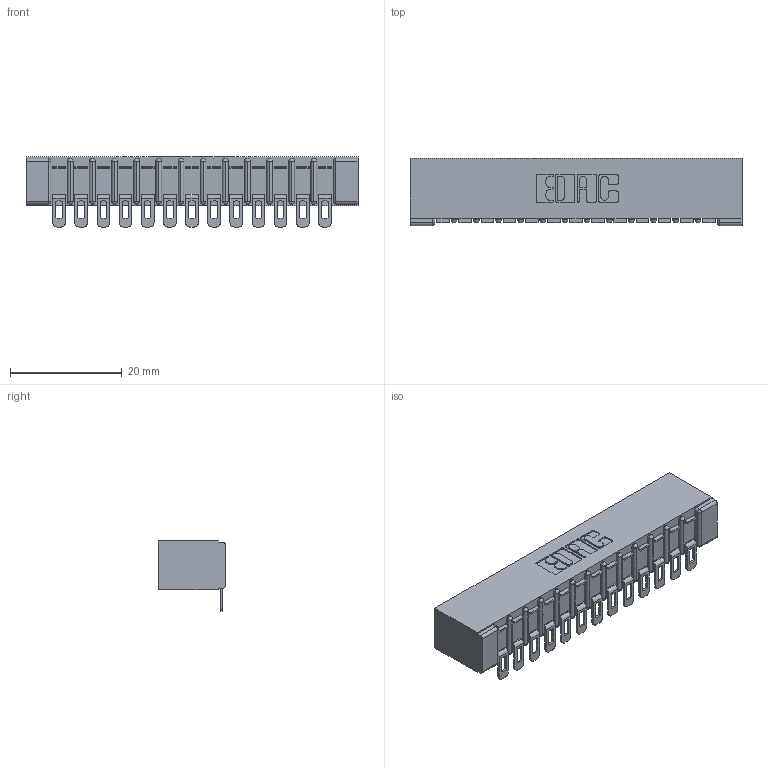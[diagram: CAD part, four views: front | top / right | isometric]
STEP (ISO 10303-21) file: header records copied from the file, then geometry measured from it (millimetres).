
FILE_DESCRIPTION (( 'STEP AP203' ), '1' );
FILE_NAME ('307-013-554-101.STEP', '2018-08-03T00:08:36', ( '' ), ( '' ), 'SwSTEP 2.0', 'SolidWorks 2016', '' );
FILE_SCHEMA (( 'CONFIG_CONTROL_DESIGN' ));
Length unit declared in the file: inch
Products named in the file (3): 307 Part_No Mounting Lugs; 307-290-002_554; 307-013-554-101
Assembly tree (14 placements, depth 2):
  307-013-554-101
    307 Part_No Mounting Lugs
    307-290-002_554  x13
Bounding box: 59.39 x 12.01 x 12.52 mm (x, y, z)
Volume: 4162.8 mm3; surface area: 7631.7 mm2
Topology: 14 solids, 14 shells, 1177 faces, 3588 edges, 2352 vertices
Faces by surface type: plane 664, cylinder 485, sphere 28
Entity records: 15407 total; most frequent: CARTESIAN_POINT 2594, ORIENTED_EDGE 2584, DIRECTION 2538, EDGE_CURVE 1292, LINE 970, VECTOR 970, VERTEX_POINT 840, AXIS2_PLACEMENT_3D 784
